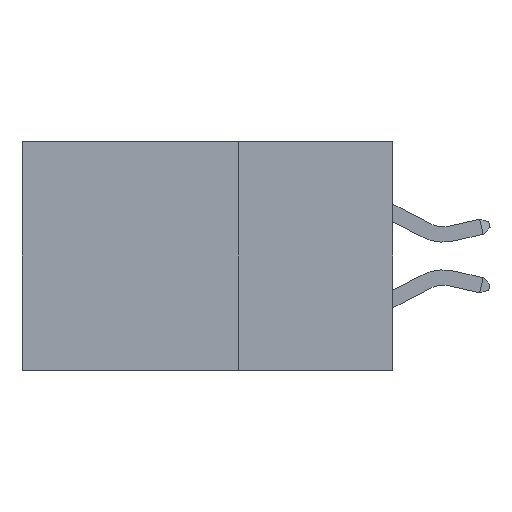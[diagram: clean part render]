
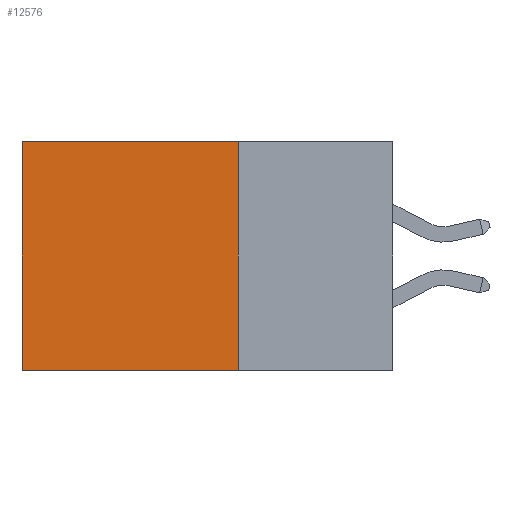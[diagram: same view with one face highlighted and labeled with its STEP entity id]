
A CAD part, left-side view. The second image highlights one B-rep face of the part: STEP entity #12576.
In plain terms, the highlighted planar face has unit normal (-1, 0, 0).
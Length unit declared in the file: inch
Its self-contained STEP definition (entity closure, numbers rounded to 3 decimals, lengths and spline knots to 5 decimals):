
#357 = CARTESIAN_POINT ( 'NONE',  ( 0.2875, 0.6, 0. ) ) ;
#645 = LINE ( 'NONE', #11208, #10070 ) ;
#1230 = EDGE_CURVE ( 'NONE', #12621, #14185, #4876, .T. ) ;
#1464 = ORIENTED_EDGE ( 'NONE', *, *, #1230, .F. ) ;
#2117 = ORIENTED_EDGE ( 'NONE', *, *, #7746, .T. ) ;
#2251 = LINE ( 'NONE', #2322, #8472 ) ;
#2322 = CARTESIAN_POINT ( 'NONE',  ( 0.2875, 0.25, 0. ) ) ;
#2442 = AXIS2_PLACEMENT_3D ( 'NONE', #6317, #14199, #7474 ) ;
#3171 = LINE ( 'NONE', #3667, #14231 ) ;
#3227 = EDGE_LOOP ( 'NONE', ( #7477, #10000, #1464, #2117 ) ) ;
#3667 = CARTESIAN_POINT ( 'NONE',  ( 0.2875, 0.25, -0.37 ) ) ;
#3955 = PLANE ( 'NONE',  #2442 ) ;
#4848 = DIRECTION ( 'NONE',  ( 0., 1., 0. ) ) ;
#4876 = LINE ( 'NONE', #12407, #13583 ) ;
#5868 = VERTEX_POINT ( 'NONE', #357 ) ;
#6167 = VERTEX_POINT ( 'NONE', #9360 ) ;
#6317 = CARTESIAN_POINT ( 'NONE',  ( 0.2875, 0.25, 0. ) ) ;
#7474 = DIRECTION ( 'NONE',  ( 0., 0., -1. ) ) ;
#7477 = ORIENTED_EDGE ( 'NONE', *, *, #14172, .T. ) ;
#7746 = EDGE_CURVE ( 'NONE', #12621, #5868, #2251, .T. ) ;
#8472 = VECTOR ( 'NONE', #10460, 39.37008 ) ;
#8690 = CARTESIAN_POINT ( 'NONE',  ( 0.2875, 0.25, 0. ) ) ;
#9039 = FACE_OUTER_BOUND ( 'NONE', #3227, .T. ) ;
#9360 = CARTESIAN_POINT ( 'NONE',  ( 0.2875, 0.6, -0.37 ) ) ;
#10000 = ORIENTED_EDGE ( 'NONE', *, *, #13831, .F. ) ;
#10070 = VECTOR ( 'NONE', #14495, 39.37008 ) ;
#10108 = CARTESIAN_POINT ( 'NONE',  ( 0.2875, 0.25, -0.37 ) ) ;
#10460 = DIRECTION ( 'NONE',  ( 0., 1., 0. ) ) ;
#11208 = CARTESIAN_POINT ( 'NONE',  ( 0.2875, 0.6, 0. ) ) ;
#12407 = CARTESIAN_POINT ( 'NONE',  ( 0.2875, 0.25, 0. ) ) ;
#12576 = ADVANCED_FACE ( 'NONE', ( #9039 ), #3955, .F. ) ;
#12621 = VERTEX_POINT ( 'NONE', #8690 ) ;
#12662 = DIRECTION ( 'NONE',  ( 0., 0., -1. ) ) ;
#13583 = VECTOR ( 'NONE', #12662, 39.37008 ) ;
#13831 = EDGE_CURVE ( 'NONE', #14185, #6167, #3171, .T. ) ;
#14172 = EDGE_CURVE ( 'NONE', #5868, #6167, #645, .T. ) ;
#14185 = VERTEX_POINT ( 'NONE', #10108 ) ;
#14199 = DIRECTION ( 'NONE',  ( 1., 0., 0. ) ) ;
#14231 = VECTOR ( 'NONE', #4848, 39.37008 ) ;
#14495 = DIRECTION ( 'NONE',  ( 0., 0., -1. ) ) ;
